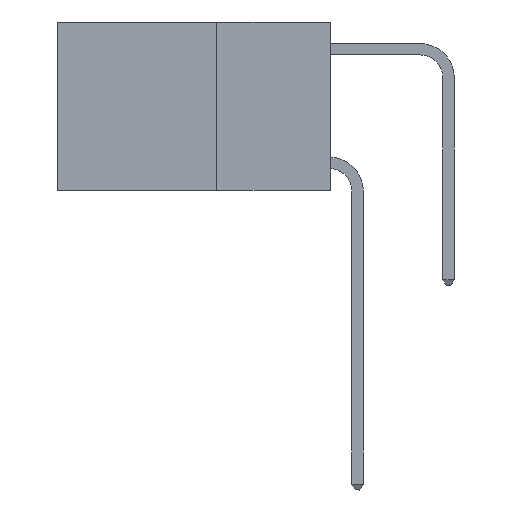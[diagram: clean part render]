
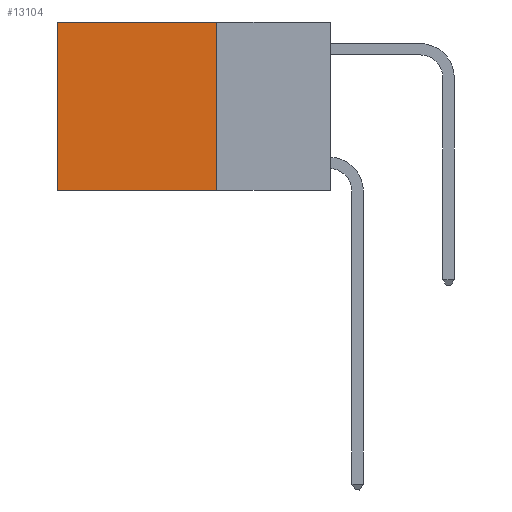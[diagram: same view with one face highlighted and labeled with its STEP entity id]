
A CAD part, left-side view. The second image highlights one B-rep face of the part: STEP entity #13104.
In plain terms, the highlighted planar face has unit normal (-1, 0, 0).
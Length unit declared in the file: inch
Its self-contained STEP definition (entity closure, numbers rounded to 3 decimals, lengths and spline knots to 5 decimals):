
#1286 = FACE_OUTER_BOUND ( 'NONE', #4714, .T. ) ;
#1746 = DIRECTION ( 'NONE',  ( 0., 0., -1. ) ) ;
#2299 = VERTEX_POINT ( 'NONE', #15826 ) ;
#2927 = CARTESIAN_POINT ( 'NONE',  ( 0.2625, 0.25, -0.37 ) ) ;
#3262 = AXIS2_PLACEMENT_3D ( 'NONE', #8139, #12479, #5120 ) ;
#3363 = CARTESIAN_POINT ( 'NONE',  ( 0.2625, 0.6, -0.37 ) ) ;
#3458 = VECTOR ( 'NONE', #15922, 39.37008 ) ;
#3890 = CARTESIAN_POINT ( 'NONE',  ( 0.2625, 0.25, 0. ) ) ;
#4240 = VERTEX_POINT ( 'NONE', #3363 ) ;
#4714 = EDGE_LOOP ( 'NONE', ( #13627, #13499, #15645, #19325 ) ) ;
#5043 = CARTESIAN_POINT ( 'NONE',  ( 0.2625, 0.25, 0. ) ) ;
#5120 = DIRECTION ( 'NONE',  ( 0., 0., -1. ) ) ;
#6875 = EDGE_CURVE ( 'NONE', #13121, #4240, #11372, .T. ) ;
#7404 = DIRECTION ( 'NONE',  ( 0., 1., 0. ) ) ;
#8139 = CARTESIAN_POINT ( 'NONE',  ( 0.2625, 0.25, 0. ) ) ;
#9100 = LINE ( 'NONE', #2927, #14305 ) ;
#11071 = VERTEX_POINT ( 'NONE', #18693 ) ;
#11169 = CARTESIAN_POINT ( 'NONE',  ( 0.2625, 0.6, 0. ) ) ;
#11372 = LINE ( 'NONE', #15225, #13713 ) ;
#11455 = LINE ( 'NONE', #3890, #3458 ) ;
#12479 = DIRECTION ( 'NONE',  ( 1., 0., 0. ) ) ;
#12571 = EDGE_CURVE ( 'NONE', #11071, #4240, #9100, .T. ) ;
#12845 = DIRECTION ( 'NONE',  ( 0., 0., -1. ) ) ;
#13104 = ADVANCED_FACE ( 'NONE', ( #1286 ), #16588, .F. ) ;
#13121 = VERTEX_POINT ( 'NONE', #11169 ) ;
#13341 = EDGE_CURVE ( 'NONE', #2299, #11071, #13716, .T. ) ;
#13499 = ORIENTED_EDGE ( 'NONE', *, *, #12571, .F. ) ;
#13627 = ORIENTED_EDGE ( 'NONE', *, *, #6875, .T. ) ;
#13713 = VECTOR ( 'NONE', #1746, 39.37008 ) ;
#13716 = LINE ( 'NONE', #5043, #15386 ) ;
#14305 = VECTOR ( 'NONE', #7404, 39.37008 ) ;
#15225 = CARTESIAN_POINT ( 'NONE',  ( 0.2625, 0.6, 0. ) ) ;
#15386 = VECTOR ( 'NONE', #12845, 39.37008 ) ;
#15645 = ORIENTED_EDGE ( 'NONE', *, *, #13341, .F. ) ;
#15826 = CARTESIAN_POINT ( 'NONE',  ( 0.2625, 0.25, 0. ) ) ;
#15922 = DIRECTION ( 'NONE',  ( 0., 1., 0. ) ) ;
#16588 = PLANE ( 'NONE',  #3262 ) ;
#17622 = EDGE_CURVE ( 'NONE', #2299, #13121, #11455, .T. ) ;
#18693 = CARTESIAN_POINT ( 'NONE',  ( 0.2625, 0.25, -0.37 ) ) ;
#19325 = ORIENTED_EDGE ( 'NONE', *, *, #17622, .T. ) ;
